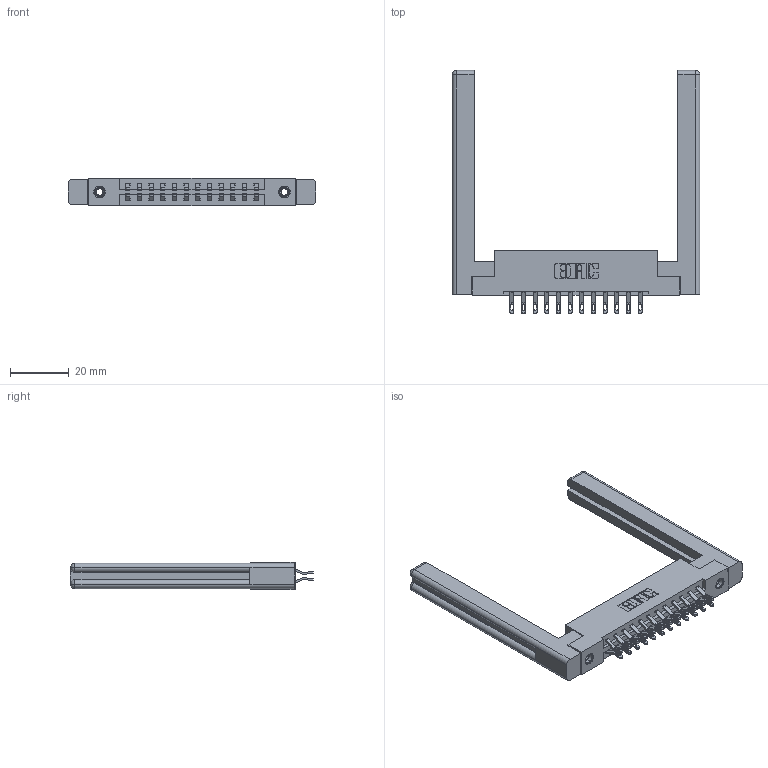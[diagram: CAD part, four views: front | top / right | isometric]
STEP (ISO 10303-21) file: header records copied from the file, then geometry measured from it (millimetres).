
FILE_DESCRIPTION (( 'STEP AP203' ), '1' );
FILE_NAME ('387-024-555-258.STEP', '2019-10-16T18:43:28', ( '' ), ( '' ), 'SwSTEP 2.0', 'SolidWorks 2016', '' );
FILE_SCHEMA (( 'CONFIG_CONTROL_DESIGN' ));
Length unit declared in the file: inch
Products named in the file (5): 307-220-058; 387-024-555-258; 345-292-001_555 Tail; 337 Part_Flush Mounting Lugs - 0.156 Dia-TI; 345-250-001_345-250-001-102
Assembly tree (29 placements, depth 2):
  387-024-555-258
    337 Part_Flush Mounting Lugs - 0.156 Dia-TI
    345-292-001_555 Tail  x24
    345-250-001_345-250-001-102  x2
    307-220-058  x2
Bounding box: 84.18 x 82.56 x 9.4 mm (x, y, z)
Volume: 15683.7 mm3; surface area: 14673.7 mm2
Topology: 29 solids, 29 shells, 1696 faces, 5201 edges, 3454 vertices
Faces by surface type: plane 1018, cylinder 654, cone 12, torus 12
Entity records: 16144 total; most frequent: CARTESIAN_POINT 2787, ORIENTED_EDGE 2632, DIRECTION 2412, EDGE_CURVE 1316, LINE 1120, VECTOR 1120, VERTEX_POINT 870, AXIS2_PLACEMENT_3D 646
